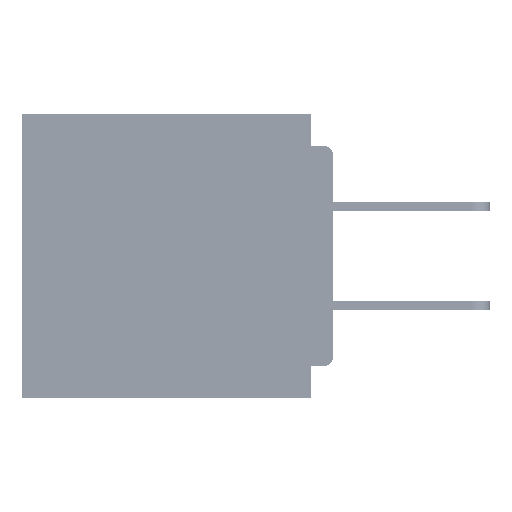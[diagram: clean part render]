
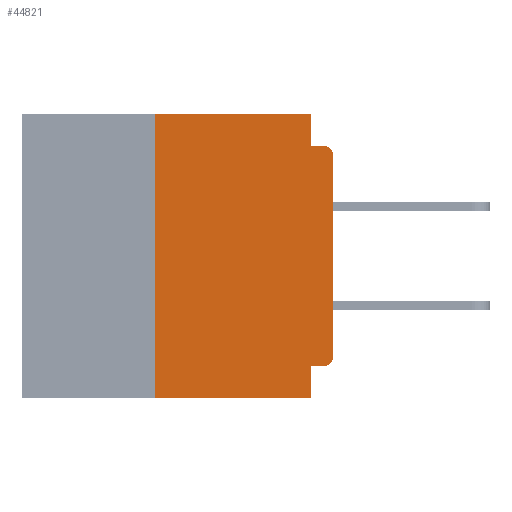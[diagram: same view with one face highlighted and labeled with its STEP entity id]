
A CAD part, left-side view. The second image highlights one B-rep face of the part: STEP entity #44821.
In plain terms, the highlighted planar face has unit normal (-1, 0, 0).
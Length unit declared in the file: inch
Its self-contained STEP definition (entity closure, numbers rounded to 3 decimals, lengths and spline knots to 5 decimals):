
#627 = CARTESIAN_POINT ( 'NONE',  ( 0., 0.031, -0.355 ) ) ;
#3704 = CARTESIAN_POINT ( 'NONE',  ( 0., 0.015, -0.045 ) ) ;
#3740 = DIRECTION ( 'NONE',  ( 1., 0., 0. ) ) ;
#3922 = CARTESIAN_POINT ( 'NONE',  ( 0., 0.25, -0.4 ) ) ;
#4572 = VECTOR ( 'NONE', #67796, 39.37008 ) ;
#5202 = CARTESIAN_POINT ( 'NONE',  ( 0., 0.031, -0.4 ) ) ;
#5282 = AXIS2_PLACEMENT_3D ( 'NONE', #19507, #3740, #40814 ) ;
#6937 = ORIENTED_EDGE ( 'NONE', *, *, #28268, .F. ) ;
#7120 = CARTESIAN_POINT ( 'NONE',  ( 0., 0., -0.34 ) ) ;
#7679 = CARTESIAN_POINT ( 'NONE',  ( 0., 0., 0. ) ) ;
#8259 = VERTEX_POINT ( 'NONE', #40014 ) ;
#9001 = DIRECTION ( 'NONE',  ( 0., 0., 1. ) ) ;
#9101 = VERTEX_POINT ( 'NONE', #36657 ) ;
#9486 = ORIENTED_EDGE ( 'NONE', *, *, #66294, .F. ) ;
#9940 = ORIENTED_EDGE ( 'NONE', *, *, #59132, .T. ) ;
#10066 = DIRECTION ( 'NONE',  ( -1., 0., 0. ) ) ;
#11752 = LINE ( 'NONE', #27781, #53968 ) ;
#13695 = EDGE_CURVE ( 'NONE', #58805, #19820, #51835, .T. ) ;
#13701 = EDGE_CURVE ( 'NONE', #63025, #51706, #64236, .T. ) ;
#14009 = VERTEX_POINT ( 'NONE', #63390 ) ;
#15552 = EDGE_CURVE ( 'NONE', #51706, #50502, #21643, .T. ) ;
#15905 = FACE_OUTER_BOUND ( 'NONE', #47639, .T. ) ;
#16837 = ORIENTED_EDGE ( 'NONE', *, *, #40983, .F. ) ;
#17701 = CARTESIAN_POINT ( 'NONE',  ( 0., 0.031, 0. ) ) ;
#18790 = VECTOR ( 'NONE', #68242, 39.37008 ) ;
#19358 = AXIS2_PLACEMENT_3D ( 'NONE', #41824, #10066, #47140 ) ;
#19492 = EDGE_CURVE ( 'NONE', #8259, #14009, #36056, .T. ) ;
#19507 = CARTESIAN_POINT ( 'NONE',  ( 0., 0.437, 0. ) ) ;
#19820 = VERTEX_POINT ( 'NONE', #33644 ) ;
#20497 = VERTEX_POINT ( 'NONE', #65212 ) ;
#20941 = ORIENTED_EDGE ( 'NONE', *, *, #26790, .T. ) ;
#21643 = LINE ( 'NONE', #65799, #46484 ) ;
#22038 = VECTOR ( 'NONE', #9001, 39.37008 ) ;
#23709 = VECTOR ( 'NONE', #34293, 39.37008 ) ;
#24017 = ORIENTED_EDGE ( 'NONE', *, *, #15552, .F. ) ;
#24650 = LINE ( 'NONE', #5202, #37106 ) ;
#24814 = PLANE ( 'NONE',  #5282 ) ;
#25052 = EDGE_CURVE ( 'NONE', #8259, #20497, #37803, .T. ) ;
#25148 = ORIENTED_EDGE ( 'NONE', *, *, #19492, .T. ) ;
#25796 = ORIENTED_EDGE ( 'NONE', *, *, #13695, .T. ) ;
#26790 = EDGE_CURVE ( 'NONE', #9101, #58805, #52500, .T. ) ;
#26802 = AXIS2_PLACEMENT_3D ( 'NONE', #28291, #65268, #33628 ) ;
#27781 = CARTESIAN_POINT ( 'NONE',  ( 0., 0.437, 0. ) ) ;
#28268 = EDGE_CURVE ( 'NONE', #9101, #35992, #46971, .T. ) ;
#28291 = CARTESIAN_POINT ( 'NONE',  ( 0., 0.015, -0.34 ) ) ;
#28835 = DIRECTION ( 'NONE',  ( 0., -1., 0. ) ) ;
#31792 = DIRECTION ( 'NONE',  ( 0., 0., -1. ) ) ;
#33628 = DIRECTION ( 'NONE',  ( 0., 0., -1. ) ) ;
#33644 = CARTESIAN_POINT ( 'NONE',  ( 0., 0., -0.06 ) ) ;
#34293 = DIRECTION ( 'NONE',  ( 0., 0., 1. ) ) ;
#35992 = VERTEX_POINT ( 'NONE', #627 ) ;
#36056 = LINE ( 'NONE', #36233, #4572 ) ;
#36233 = CARTESIAN_POINT ( 'NONE',  ( 0., 0.437, -0.4 ) ) ;
#36657 = CARTESIAN_POINT ( 'NONE',  ( 0., 0.015, -0.355 ) ) ;
#36725 = ORIENTED_EDGE ( 'NONE', *, *, #25052, .F. ) ;
#37106 = VECTOR ( 'NONE', #31792, 39.37008 ) ;
#37803 = LINE ( 'NONE', #3922, #22038 ) ;
#40014 = CARTESIAN_POINT ( 'NONE',  ( 0., 0.25, -0.4 ) ) ;
#40814 = DIRECTION ( 'NONE',  ( 0., 0., -1. ) ) ;
#40983 = EDGE_CURVE ( 'NONE', #35992, #14009, #24650, .T. ) ;
#41824 = CARTESIAN_POINT ( 'NONE',  ( 0., 0.015, -0.06 ) ) ;
#44821 = ADVANCED_FACE ( 'NONE', ( #15905 ), #24814, .F. ) ;
#44976 = DIRECTION ( 'NONE',  ( 0., 0., -1. ) ) ;
#46484 = VECTOR ( 'NONE', #28835, 39.37008 ) ;
#46971 = LINE ( 'NONE', #63023, #18790 ) ;
#47140 = DIRECTION ( 'NONE',  ( 0., 0., -1. ) ) ;
#47639 = EDGE_LOOP ( 'NONE', ( #25796, #9940, #24017, #60017, #9486, #36725, #25148, #16837, #6937, #20941 ) ) ;
#50039 = CARTESIAN_POINT ( 'NONE',  ( 0., 0.031, 0. ) ) ;
#50188 = VECTOR ( 'NONE', #44976, 39.37008 ) ;
#50502 = VERTEX_POINT ( 'NONE', #3704 ) ;
#51706 = VERTEX_POINT ( 'NONE', #66662 ) ;
#51835 = LINE ( 'NONE', #7679, #23709 ) ;
#52500 = CIRCLE ( 'NONE', #26802, 0.015 ) ;
#53968 = VECTOR ( 'NONE', #59473, 39.37008 ) ;
#54079 = CIRCLE ( 'NONE', #19358, 0.015 ) ;
#58805 = VERTEX_POINT ( 'NONE', #7120 ) ;
#59132 = EDGE_CURVE ( 'NONE', #19820, #50502, #54079, .T. ) ;
#59473 = DIRECTION ( 'NONE',  ( 0., -1., 0. ) ) ;
#60017 = ORIENTED_EDGE ( 'NONE', *, *, #13701, .F. ) ;
#63023 = CARTESIAN_POINT ( 'NONE',  ( 0., 0., -0.355 ) ) ;
#63025 = VERTEX_POINT ( 'NONE', #17701 ) ;
#63390 = CARTESIAN_POINT ( 'NONE',  ( 0., 0.031, -0.4 ) ) ;
#64236 = LINE ( 'NONE', #50039, #50188 ) ;
#65212 = CARTESIAN_POINT ( 'NONE',  ( 0., 0.25, 0. ) ) ;
#65268 = DIRECTION ( 'NONE',  ( -1., 0., 0. ) ) ;
#65799 = CARTESIAN_POINT ( 'NONE',  ( 0., 0., -0.045 ) ) ;
#66294 = EDGE_CURVE ( 'NONE', #20497, #63025, #11752, .T. ) ;
#66662 = CARTESIAN_POINT ( 'NONE',  ( 0., 0.031, -0.045 ) ) ;
#67796 = DIRECTION ( 'NONE',  ( 0., -1., 0. ) ) ;
#68242 = DIRECTION ( 'NONE',  ( 0., 1., 0. ) ) ;
